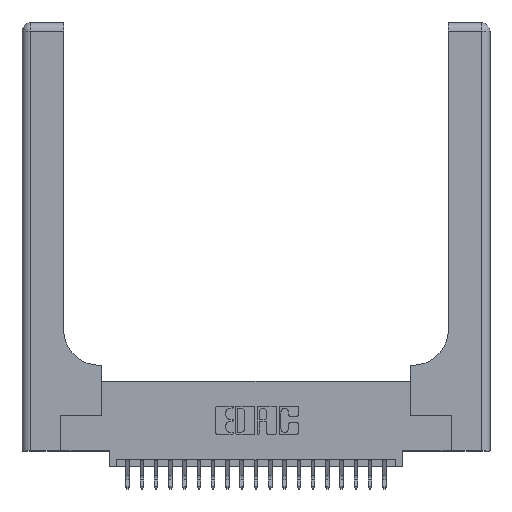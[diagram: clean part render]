
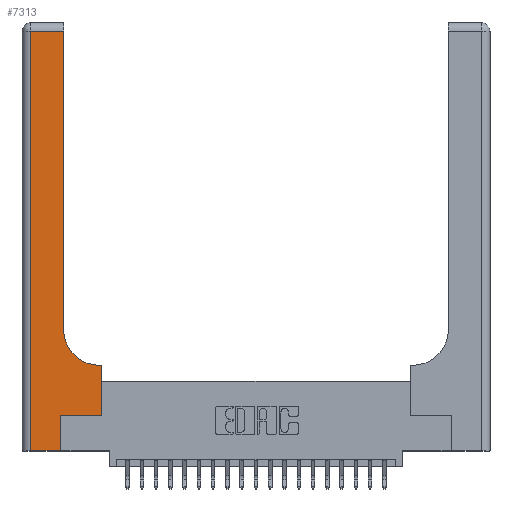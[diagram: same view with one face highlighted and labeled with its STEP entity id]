
A CAD part, top view. The second image highlights one B-rep face of the part: STEP entity #7313.
In plain terms, the highlighted planar face has unit normal (0, 0, 1).
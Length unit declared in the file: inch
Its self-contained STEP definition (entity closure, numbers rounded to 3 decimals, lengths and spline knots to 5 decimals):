
#751 = LINE ( 'NONE', #13033, #15877 ) ;
#955 = FACE_OUTER_BOUND ( 'NONE', #10303, .T. ) ;
#1006 = VERTEX_POINT ( 'NONE', #7060 ) ;
#1265 = VECTOR ( 'NONE', #17023, 39.37008 ) ;
#1598 = VERTEX_POINT ( 'NONE', #16107 ) ;
#1751 = VECTOR ( 'NONE', #3717, 39.37008 ) ;
#2086 = CARTESIAN_POINT ( 'NONE',  ( 0., 2.94, 0.37 ) ) ;
#2402 = ORIENTED_EDGE ( 'NONE', *, *, #5989, .T. ) ;
#2537 = ORIENTED_EDGE ( 'NONE', *, *, #9247, .T. ) ;
#3224 = ORIENTED_EDGE ( 'NONE', *, *, #15407, .T. ) ;
#3301 = CIRCLE ( 'NONE', #12752, 0.25 ) ;
#3717 = DIRECTION ( 'NONE',  ( 0., -1., 0. ) ) ;
#3968 = VERTEX_POINT ( 'NONE', #8495 ) ;
#4491 = ORIENTED_EDGE ( 'NONE', *, *, #13817, .T. ) ;
#4810 = DIRECTION ( 'NONE',  ( 0., 1., 0. ) ) ;
#4909 = CARTESIAN_POINT ( 'NONE',  ( 0.5585, 0.25, 0.37 ) ) ;
#5010 = ORIENTED_EDGE ( 'NONE', *, *, #15056, .T. ) ;
#5269 = DIRECTION ( 'NONE',  ( -1., 0., 0. ) ) ;
#5693 = CARTESIAN_POINT ( 'NONE',  ( 0.2915, 2.94, 0.37 ) ) ;
#5873 = LINE ( 'NONE', #19554, #17209 ) ;
#5989 = EDGE_CURVE ( 'NONE', #20203, #10943, #751, .T. ) ;
#6646 = DIRECTION ( 'NONE',  ( 0., 1., 0. ) ) ;
#7060 = CARTESIAN_POINT ( 'NONE',  ( 0.269, 0., 0.37 ) ) ;
#7103 = DIRECTION ( 'NONE',  ( 0., 0., -1. ) ) ;
#7233 = LINE ( 'NONE', #23571, #1751 ) ;
#7313 = ADVANCED_FACE ( 'NONE', ( #955 ), #16212, .F. ) ;
#7355 = EDGE_CURVE ( 'NONE', #1598, #8285, #19762, .T. ) ;
#7736 = EDGE_CURVE ( 'NONE', #9666, #1006, #12102, .T. ) ;
#8285 = VERTEX_POINT ( 'NONE', #4909 ) ;
#8451 = EDGE_CURVE ( 'NONE', #10943, #3968, #19407, .T. ) ;
#8495 = CARTESIAN_POINT ( 'NONE',  ( 0.06, 2.94, 0.37 ) ) ;
#9247 = EDGE_CURVE ( 'NONE', #16353, #11222, #19952, .T. ) ;
#9666 = VERTEX_POINT ( 'NONE', #14838 ) ;
#10303 = EDGE_LOOP ( 'NONE', ( #2402, #15044, #5010, #22327, #3224, #16847, #14156, #2537, #4491 ) ) ;
#10832 = DIRECTION ( 'NONE',  ( 1., 0., 0. ) ) ;
#10943 = VERTEX_POINT ( 'NONE', #5693 ) ;
#11222 = VERTEX_POINT ( 'NONE', #19480 ) ;
#11261 = AXIS2_PLACEMENT_3D ( 'NONE', #19938, #7103, #5269 ) ;
#11557 = CARTESIAN_POINT ( 'NONE',  ( 0.269, 0., 0.37 ) ) ;
#11778 = DIRECTION ( 'NONE',  ( -1., 0., 0. ) ) ;
#12102 = LINE ( 'NONE', #20997, #13523 ) ;
#12514 = CARTESIAN_POINT ( 'NONE',  ( 0.269, 0.25, 0.37 ) ) ;
#12752 = AXIS2_PLACEMENT_3D ( 'NONE', #23402, #14317, #21674 ) ;
#13033 = CARTESIAN_POINT ( 'NONE',  ( 0.2915, 3., 0.37 ) ) ;
#13262 = LINE ( 'NONE', #11557, #1265 ) ;
#13523 = VECTOR ( 'NONE', #15632, 39.37008 ) ;
#13817 = EDGE_CURVE ( 'NONE', #11222, #20203, #3301, .T. ) ;
#14156 = ORIENTED_EDGE ( 'NONE', *, *, #21528, .T. ) ;
#14317 = DIRECTION ( 'NONE',  ( 0., 0., -1. ) ) ;
#14838 = CARTESIAN_POINT ( 'NONE',  ( 0.06, 0., 0.37 ) ) ;
#14850 = DIRECTION ( 'NONE',  ( -1., 0., 0. ) ) ;
#14970 = VECTOR ( 'NONE', #10832, 39.37008 ) ;
#15044 = ORIENTED_EDGE ( 'NONE', *, *, #8451, .T. ) ;
#15056 = EDGE_CURVE ( 'NONE', #3968, #9666, #7233, .T. ) ;
#15189 = VECTOR ( 'NONE', #14850, 39.37008 ) ;
#15407 = EDGE_CURVE ( 'NONE', #1006, #1598, #13262, .T. ) ;
#15632 = DIRECTION ( 'NONE',  ( 1., 0., 0. ) ) ;
#15877 = VECTOR ( 'NONE', #4810, 39.37008 ) ;
#16107 = CARTESIAN_POINT ( 'NONE',  ( 0.269, 0.25, 0.37 ) ) ;
#16212 = PLANE ( 'NONE',  #11261 ) ;
#16353 = VERTEX_POINT ( 'NONE', #17278 ) ;
#16813 = VECTOR ( 'NONE', #11778, 39.37008 ) ;
#16847 = ORIENTED_EDGE ( 'NONE', *, *, #7355, .T. ) ;
#17023 = DIRECTION ( 'NONE',  ( 0., 1., 0. ) ) ;
#17209 = VECTOR ( 'NONE', #6646, 39.37008 ) ;
#17278 = CARTESIAN_POINT ( 'NONE',  ( 0.5585, 0.6, 0.37 ) ) ;
#19407 = LINE ( 'NONE', #2086, #15189 ) ;
#19480 = CARTESIAN_POINT ( 'NONE',  ( 0.5415, 0.6, 0.37 ) ) ;
#19554 = CARTESIAN_POINT ( 'NONE',  ( 0.5585, 0.25, 0.37 ) ) ;
#19762 = LINE ( 'NONE', #12514, #14970 ) ;
#19938 = CARTESIAN_POINT ( 'NONE',  ( 0., 3., 0.37 ) ) ;
#19952 = LINE ( 'NONE', #22625, #16813 ) ;
#20203 = VERTEX_POINT ( 'NONE', #20229 ) ;
#20229 = CARTESIAN_POINT ( 'NONE',  ( 0.2915, 0.85, 0.37 ) ) ;
#20997 = CARTESIAN_POINT ( 'NONE',  ( 0., 0., 0.37 ) ) ;
#21528 = EDGE_CURVE ( 'NONE', #8285, #16353, #5873, .T. ) ;
#21674 = DIRECTION ( 'NONE',  ( 1., 0., 0. ) ) ;
#22327 = ORIENTED_EDGE ( 'NONE', *, *, #7736, .T. ) ;
#22625 = CARTESIAN_POINT ( 'NONE',  ( 0.2915, 0.6, 0.37 ) ) ;
#23402 = CARTESIAN_POINT ( 'NONE',  ( 0.5415, 0.85, 0.37 ) ) ;
#23571 = CARTESIAN_POINT ( 'NONE',  ( 0.06, 3., 0.37 ) ) ;
